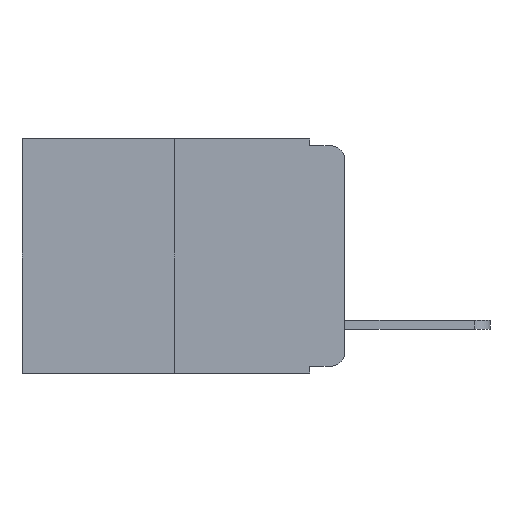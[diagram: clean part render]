
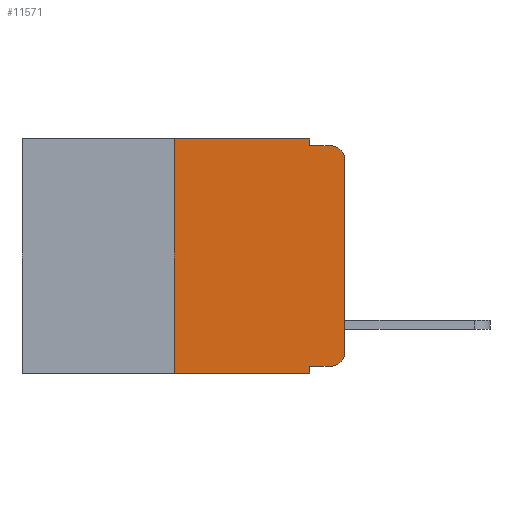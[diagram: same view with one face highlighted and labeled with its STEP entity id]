
A CAD part, left-side view. The second image highlights one B-rep face of the part: STEP entity #11571.
In plain terms, the highlighted planar face has unit normal (-1, 0, 0).
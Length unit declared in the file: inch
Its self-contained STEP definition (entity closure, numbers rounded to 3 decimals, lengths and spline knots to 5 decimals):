
#74 = VERTEX_POINT ( 'NONE', #5082 ) ;
#528 = CARTESIAN_POINT ( 'NONE',  ( 0., 0., -0.03 ) ) ;
#890 = DIRECTION ( 'NONE',  ( -1., 0., 0. ) ) ;
#1043 = VECTOR ( 'NONE', #4532, 39.37008 ) ;
#1475 = ORIENTED_EDGE ( 'NONE', *, *, #9441, .T. ) ;
#1677 = CARTESIAN_POINT ( 'NONE',  ( 0., 0.473, 0. ) ) ;
#2156 = DIRECTION ( 'NONE',  ( 0., 0., -1. ) ) ;
#2507 = LINE ( 'NONE', #15145, #8935 ) ;
#2625 = CARTESIAN_POINT ( 'NONE',  ( 0., 0.051, -0.333 ) ) ;
#2659 = ORIENTED_EDGE ( 'NONE', *, *, #6845, .F. ) ;
#2703 = CARTESIAN_POINT ( 'NONE',  ( 0., 0.051, -0.01 ) ) ;
#2944 = CARTESIAN_POINT ( 'NONE',  ( 0., 0.051, -0.343 ) ) ;
#2984 = CARTESIAN_POINT ( 'NONE',  ( 0., 0.051, -0.333 ) ) ;
#3029 = FACE_OUTER_BOUND ( 'NONE', #10923, .T. ) ;
#3095 = ORIENTED_EDGE ( 'NONE', *, *, #13882, .T. ) ;
#3113 = DIRECTION ( 'NONE',  ( 1., 0., 0. ) ) ;
#3339 = DIRECTION ( 'NONE',  ( 0., 0., -1. ) ) ;
#3397 = CARTESIAN_POINT ( 'NONE',  ( 0., 0.051, -0.01 ) ) ;
#3462 = VERTEX_POINT ( 'NONE', #2984 ) ;
#3473 = ORIENTED_EDGE ( 'NONE', *, *, #13451, .F. ) ;
#3577 = LINE ( 'NONE', #2625, #6197 ) ;
#3862 = VERTEX_POINT ( 'NONE', #5141 ) ;
#4056 = DIRECTION ( 'NONE',  ( 0., 0., 1. ) ) ;
#4084 = VERTEX_POINT ( 'NONE', #2703 ) ;
#4168 = VERTEX_POINT ( 'NONE', #528 ) ;
#4252 = VERTEX_POINT ( 'NONE', #7466 ) ;
#4385 = AXIS2_PLACEMENT_3D ( 'NONE', #8556, #890, #2156 ) ;
#4532 = DIRECTION ( 'NONE',  ( 0., -1., 0. ) ) ;
#4676 = CARTESIAN_POINT ( 'NONE',  ( 0., 0.25, 0. ) ) ;
#4689 = CIRCLE ( 'NONE', #6589, 0.02 ) ;
#4798 = VECTOR ( 'NONE', #7358, 39.37008 ) ;
#5082 = CARTESIAN_POINT ( 'NONE',  ( 0., 0.25, -0.343 ) ) ;
#5141 = CARTESIAN_POINT ( 'NONE',  ( 0., 0.051, 0. ) ) ;
#5290 = ORIENTED_EDGE ( 'NONE', *, *, #10569, .T. ) ;
#5523 = VECTOR ( 'NONE', #4056, 39.37008 ) ;
#6197 = VECTOR ( 'NONE', #11599, 39.37008 ) ;
#6589 = AXIS2_PLACEMENT_3D ( 'NONE', #9895, #8417, #11213 ) ;
#6642 = CARTESIAN_POINT ( 'NONE',  ( 0., 0.051, 0. ) ) ;
#6653 = ORIENTED_EDGE ( 'NONE', *, *, #7406, .T. ) ;
#6845 = EDGE_CURVE ( 'NONE', #3462, #11455, #13003, .T. ) ;
#7130 = CARTESIAN_POINT ( 'NONE',  ( 0., 0.473, -0.343 ) ) ;
#7358 = DIRECTION ( 'NONE',  ( 0., -1., 0. ) ) ;
#7406 = EDGE_CURVE ( 'NONE', #74, #11455, #10393, .T. ) ;
#7466 = CARTESIAN_POINT ( 'NONE',  ( 0., 0., -0.313 ) ) ;
#7742 = ORIENTED_EDGE ( 'NONE', *, *, #15672, .F. ) ;
#7798 = DIRECTION ( 'NONE',  ( 0., 0., -1. ) ) ;
#7873 = VECTOR ( 'NONE', #7798, 39.37008 ) ;
#8207 = PLANE ( 'NONE',  #10015 ) ;
#8254 = ORIENTED_EDGE ( 'NONE', *, *, #11572, .F. ) ;
#8417 = DIRECTION ( 'NONE',  ( -1., 0., 0. ) ) ;
#8497 = LINE ( 'NONE', #10495, #5523 ) ;
#8556 = CARTESIAN_POINT ( 'NONE',  ( 0., 0.02, -0.03 ) ) ;
#8935 = VECTOR ( 'NONE', #13791, 39.37008 ) ;
#9369 = DIRECTION ( 'NONE',  ( 0., 0., -1. ) ) ;
#9441 = EDGE_CURVE ( 'NONE', #4252, #4168, #8497, .T. ) ;
#9895 = CARTESIAN_POINT ( 'NONE',  ( 0., 0.02, -0.313 ) ) ;
#10015 = AXIS2_PLACEMENT_3D ( 'NONE', #10809, #3113, #3339 ) ;
#10393 = LINE ( 'NONE', #7130, #4798 ) ;
#10495 = CARTESIAN_POINT ( 'NONE',  ( 0., 0., 0. ) ) ;
#10569 = EDGE_CURVE ( 'NONE', #12898, #4252, #4689, .T. ) ;
#10809 = CARTESIAN_POINT ( 'NONE',  ( 0., 0.473, 0. ) ) ;
#10923 = EDGE_LOOP ( 'NONE', ( #1475, #13334, #8254, #14164, #3473, #7742, #6653, #2659, #3095, #5290 ) ) ;
#11126 = CIRCLE ( 'NONE', #4385, 0.02 ) ;
#11201 = CARTESIAN_POINT ( 'NONE',  ( 0., 0.02, -0.333 ) ) ;
#11213 = DIRECTION ( 'NONE',  ( 0., 0., -1. ) ) ;
#11353 = EDGE_CURVE ( 'NONE', #3862, #4084, #15284, .T. ) ;
#11455 = VERTEX_POINT ( 'NONE', #2944 ) ;
#11571 = ADVANCED_FACE ( 'NONE', ( #3029 ), #8207, .F. ) ;
#11572 = EDGE_CURVE ( 'NONE', #4084, #12847, #13465, .T. ) ;
#11599 = DIRECTION ( 'NONE',  ( 0., -1., 0. ) ) ;
#11930 = CARTESIAN_POINT ( 'NONE',  ( 0., 0.051, 0. ) ) ;
#12059 = DIRECTION ( 'NONE',  ( 0., -1., 0. ) ) ;
#12271 = VERTEX_POINT ( 'NONE', #4676 ) ;
#12847 = VERTEX_POINT ( 'NONE', #15858 ) ;
#12898 = VERTEX_POINT ( 'NONE', #11201 ) ;
#12997 = LINE ( 'NONE', #1677, #16214 ) ;
#13003 = LINE ( 'NONE', #11930, #14405 ) ;
#13334 = ORIENTED_EDGE ( 'NONE', *, *, #15952, .T. ) ;
#13451 = EDGE_CURVE ( 'NONE', #12271, #3862, #12997, .T. ) ;
#13465 = LINE ( 'NONE', #3397, #1043 ) ;
#13791 = DIRECTION ( 'NONE',  ( 0., 0., 1. ) ) ;
#13882 = EDGE_CURVE ( 'NONE', #3462, #12898, #3577, .T. ) ;
#14164 = ORIENTED_EDGE ( 'NONE', *, *, #11353, .F. ) ;
#14405 = VECTOR ( 'NONE', #9369, 39.37008 ) ;
#15145 = CARTESIAN_POINT ( 'NONE',  ( 0., 0.25, 0. ) ) ;
#15284 = LINE ( 'NONE', #6642, #7873 ) ;
#15672 = EDGE_CURVE ( 'NONE', #74, #12271, #2507, .T. ) ;
#15858 = CARTESIAN_POINT ( 'NONE',  ( 0., 0.02, -0.01 ) ) ;
#15952 = EDGE_CURVE ( 'NONE', #4168, #12847, #11126, .T. ) ;
#16214 = VECTOR ( 'NONE', #12059, 39.37008 ) ;
